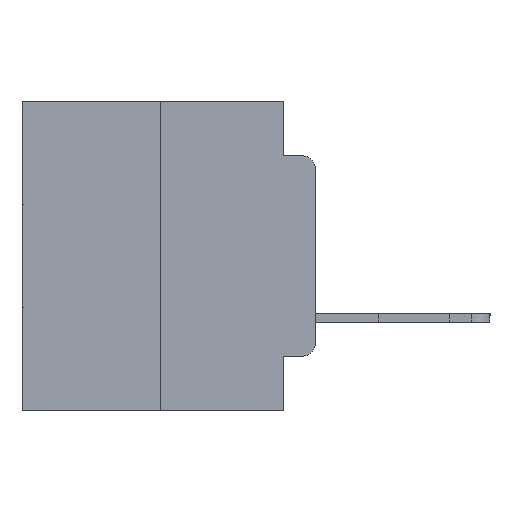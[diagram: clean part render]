
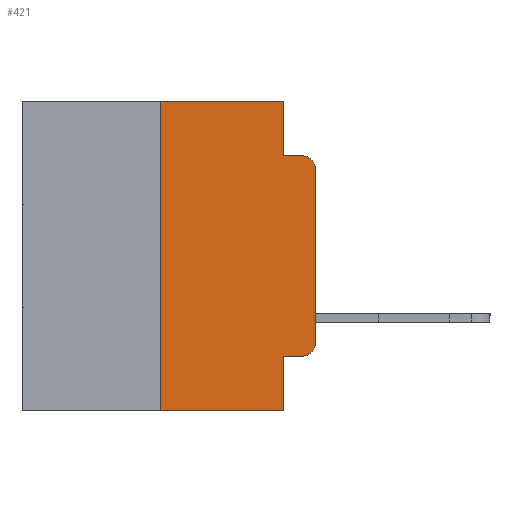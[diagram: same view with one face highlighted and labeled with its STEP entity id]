
A CAD part, left-side view. The second image highlights one B-rep face of the part: STEP entity #421.
In plain terms, the highlighted planar face has unit normal (-1, 0, 0).
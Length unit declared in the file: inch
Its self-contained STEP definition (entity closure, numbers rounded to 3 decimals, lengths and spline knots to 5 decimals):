
#283 = DIRECTION ( 'NONE',  ( 0., 0., -1. ) ) ;
#295 = DIRECTION ( 'NONE',  ( 0., 0., -1. ) ) ;
#421 = ADVANCED_FACE ( 'NONE', ( #17528 ), #1549, .F. ) ;
#489 = DIRECTION ( 'NONE',  ( 0., 0., -1. ) ) ;
#713 = DIRECTION ( 'NONE',  ( 0., -1., 0. ) ) ;
#795 = VERTEX_POINT ( 'NONE', #12079 ) ;
#1243 = VERTEX_POINT ( 'NONE', #7440 ) ;
#1549 = PLANE ( 'NONE',  #17860 ) ;
#3015 = VERTEX_POINT ( 'NONE', #20187 ) ;
#4128 = VECTOR ( 'NONE', #19859, 39.37008 ) ;
#4221 = LINE ( 'NONE', #12362, #19670 ) ;
#4393 = LINE ( 'NONE', #13563, #20469 ) ;
#5567 = ORIENTED_EDGE ( 'NONE', *, *, #7437, .F. ) ;
#6195 = CARTESIAN_POINT ( 'NONE',  ( 0., 0.051, -0.5 ) ) ;
#6582 = ORIENTED_EDGE ( 'NONE', *, *, #16401, .T. ) ;
#6792 = DIRECTION ( 'NONE',  ( 0., 0., 1. ) ) ;
#6961 = LINE ( 'NONE', #8995, #22149 ) ;
#7437 = EDGE_CURVE ( 'NONE', #18281, #8223, #20866, .T. ) ;
#7440 = CARTESIAN_POINT ( 'NONE',  ( 0., 0., -0.3915 ) ) ;
#8223 = VERTEX_POINT ( 'NONE', #26387 ) ;
#8995 = CARTESIAN_POINT ( 'NONE',  ( 0., 0.051, 0. ) ) ;
#9496 = LINE ( 'NONE', #11836, #24341 ) ;
#9609 = CARTESIAN_POINT ( 'NONE',  ( 0., 0.473, 0. ) ) ;
#9989 = AXIS2_PLACEMENT_3D ( 'NONE', #25324, #13549, #283 ) ;
#10097 = ORIENTED_EDGE ( 'NONE', *, *, #23081, .T. ) ;
#10433 = ORIENTED_EDGE ( 'NONE', *, *, #15081, .T. ) ;
#10734 = VERTEX_POINT ( 'NONE', #6195 ) ;
#11698 = CARTESIAN_POINT ( 'NONE',  ( 0., 0.051, -0.0885 ) ) ;
#11836 = CARTESIAN_POINT ( 'NONE',  ( 0., 0.051, -0.4115 ) ) ;
#12079 = CARTESIAN_POINT ( 'NONE',  ( 0., 0.051, -0.4115 ) ) ;
#12362 = CARTESIAN_POINT ( 'NONE',  ( 0., 0.473, -0.5 ) ) ;
#12407 = CARTESIAN_POINT ( 'NONE',  ( 0., 0.02, -0.4115 ) ) ;
#12815 = ORIENTED_EDGE ( 'NONE', *, *, #21742, .F. ) ;
#13549 = DIRECTION ( 'NONE',  ( -1., 0., 0. ) ) ;
#13563 = CARTESIAN_POINT ( 'NONE',  ( 0., 0.051, 0. ) ) ;
#13741 = DIRECTION ( 'NONE',  ( -1., 0., 0. ) ) ;
#13971 = VERTEX_POINT ( 'NONE', #11698 ) ;
#14035 = CARTESIAN_POINT ( 'NONE',  ( 0., 0.02, -0.0885 ) ) ;
#14105 = VERTEX_POINT ( 'NONE', #14035 ) ;
#14783 = AXIS2_PLACEMENT_3D ( 'NONE', #25478, #13741, #489 ) ;
#14865 = VECTOR ( 'NONE', #24355, 39.37008 ) ;
#14878 = CIRCLE ( 'NONE', #14783, 0.02 ) ;
#15081 = EDGE_CURVE ( 'NONE', #22789, #1243, #25019, .T. ) ;
#16401 = EDGE_CURVE ( 'NONE', #795, #22789, #9496, .T. ) ;
#16786 = CARTESIAN_POINT ( 'NONE',  ( 0., 0.25, 0. ) ) ;
#16839 = ORIENTED_EDGE ( 'NONE', *, *, #19037, .F. ) ;
#16850 = CARTESIAN_POINT ( 'NONE',  ( 0., 0.25, 0. ) ) ;
#17100 = LINE ( 'NONE', #16850, #21789 ) ;
#17408 = EDGE_CURVE ( 'NONE', #3015, #10734, #4221, .T. ) ;
#17528 = FACE_OUTER_BOUND ( 'NONE', #24420, .T. ) ;
#17710 = EDGE_CURVE ( 'NONE', #795, #10734, #6961, .T. ) ;
#17735 = ORIENTED_EDGE ( 'NONE', *, *, #17408, .T. ) ;
#17860 = AXIS2_PLACEMENT_3D ( 'NONE', #22352, #26573, #26490 ) ;
#18281 = VERTEX_POINT ( 'NONE', #16786 ) ;
#18359 = DIRECTION ( 'NONE',  ( 0., -1., 0. ) ) ;
#19037 = EDGE_CURVE ( 'NONE', #3015, #18281, #17100, .T. ) ;
#19670 = VECTOR ( 'NONE', #18359, 39.37008 ) ;
#19676 = CARTESIAN_POINT ( 'NONE',  ( 0., 0., -0.1085 ) ) ;
#19859 = DIRECTION ( 'NONE',  ( 0., -1., 0. ) ) ;
#20187 = CARTESIAN_POINT ( 'NONE',  ( 0., 0.25, -0.5 ) ) ;
#20397 = EDGE_CURVE ( 'NONE', #8223, #13971, #4393, .T. ) ;
#20408 = VECTOR ( 'NONE', #6792, 39.37008 ) ;
#20417 = CARTESIAN_POINT ( 'NONE',  ( 0., 0.051, -0.0885 ) ) ;
#20469 = VECTOR ( 'NONE', #295, 39.37008 ) ;
#20866 = LINE ( 'NONE', #9609, #4128 ) ;
#21030 = LINE ( 'NONE', #21214, #20408 ) ;
#21214 = CARTESIAN_POINT ( 'NONE',  ( 0., 0., 0. ) ) ;
#21742 = EDGE_CURVE ( 'NONE', #13971, #14105, #25293, .T. ) ;
#21789 = VECTOR ( 'NONE', #26534, 39.37008 ) ;
#22149 = VECTOR ( 'NONE', #25118, 39.37008 ) ;
#22352 = CARTESIAN_POINT ( 'NONE',  ( 0., 0.473, 0. ) ) ;
#22430 = ORIENTED_EDGE ( 'NONE', *, *, #17710, .F. ) ;
#22789 = VERTEX_POINT ( 'NONE', #12407 ) ;
#23081 = EDGE_CURVE ( 'NONE', #23952, #14105, #14878, .T. ) ;
#23952 = VERTEX_POINT ( 'NONE', #19676 ) ;
#23973 = ORIENTED_EDGE ( 'NONE', *, *, #20397, .F. ) ;
#24341 = VECTOR ( 'NONE', #713, 39.37008 ) ;
#24343 = EDGE_CURVE ( 'NONE', #1243, #23952, #21030, .T. ) ;
#24355 = DIRECTION ( 'NONE',  ( 0., -1., 0. ) ) ;
#24420 = EDGE_LOOP ( 'NONE', ( #25988, #10097, #12815, #23973, #5567, #16839, #17735, #22430, #6582, #10433 ) ) ;
#25019 = CIRCLE ( 'NONE', #9989, 0.02 ) ;
#25118 = DIRECTION ( 'NONE',  ( 0., 0., -1. ) ) ;
#25293 = LINE ( 'NONE', #20417, #14865 ) ;
#25324 = CARTESIAN_POINT ( 'NONE',  ( 0., 0.02, -0.3915 ) ) ;
#25478 = CARTESIAN_POINT ( 'NONE',  ( 0., 0.02, -0.1085 ) ) ;
#25988 = ORIENTED_EDGE ( 'NONE', *, *, #24343, .T. ) ;
#26387 = CARTESIAN_POINT ( 'NONE',  ( 0., 0.051, 0. ) ) ;
#26490 = DIRECTION ( 'NONE',  ( 0., 0., -1. ) ) ;
#26534 = DIRECTION ( 'NONE',  ( 0., 0., 1. ) ) ;
#26573 = DIRECTION ( 'NONE',  ( 1., 0., 0. ) ) ;
